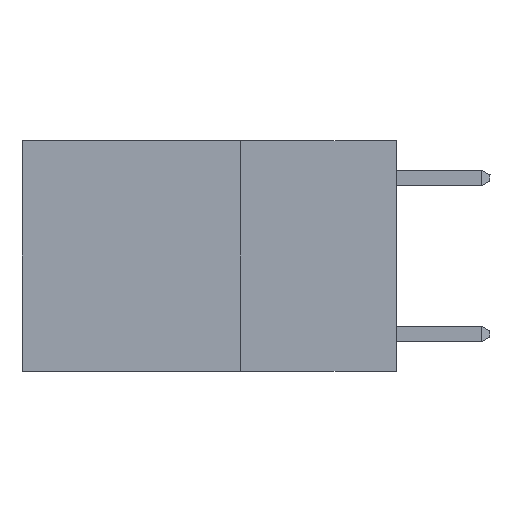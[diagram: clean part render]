
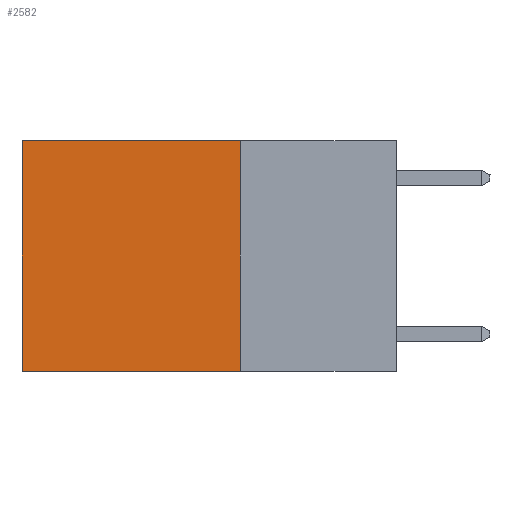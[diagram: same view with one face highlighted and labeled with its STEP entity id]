
A CAD part, left-side view. The second image highlights one B-rep face of the part: STEP entity #2582.
In plain terms, the highlighted planar face has unit normal (-1, 0, 0).
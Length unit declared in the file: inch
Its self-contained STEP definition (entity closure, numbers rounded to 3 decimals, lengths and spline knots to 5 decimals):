
#59 = LINE ( 'NONE', #6699, #10826 ) ;
#206 = CARTESIAN_POINT ( 'NONE',  ( 0.2625, 0.25, -0.37 ) ) ;
#1001 = DIRECTION ( 'NONE',  ( 0., 1., 0. ) ) ;
#1165 = CARTESIAN_POINT ( 'NONE',  ( 0.2625, 0.25, 0. ) ) ;
#1346 = EDGE_CURVE ( 'NONE', #12478, #9036, #5121, .T. ) ;
#1813 = CARTESIAN_POINT ( 'NONE',  ( 0.2625, 0.25, 0. ) ) ;
#2383 = VECTOR ( 'NONE', #9226, 39.37008 ) ;
#2495 = ORIENTED_EDGE ( 'NONE', *, *, #9617, .F. ) ;
#2582 = ADVANCED_FACE ( 'NONE', ( #8366 ), #13596, .F. ) ;
#3487 = EDGE_CURVE ( 'NONE', #10456, #3596, #10041, .T. ) ;
#3596 = VERTEX_POINT ( 'NONE', #206 ) ;
#3707 = LINE ( 'NONE', #1165, #13498 ) ;
#4572 = ORIENTED_EDGE ( 'NONE', *, *, #15252, .T. ) ;
#4646 = EDGE_LOOP ( 'NONE', ( #11900, #2495, #7291, #4572 ) ) ;
#5121 = LINE ( 'NONE', #14393, #2383 ) ;
#6699 = CARTESIAN_POINT ( 'NONE',  ( 0.2625, 0.25, -0.37 ) ) ;
#7075 = DIRECTION ( 'NONE',  ( 1., 0., 0. ) ) ;
#7291 = ORIENTED_EDGE ( 'NONE', *, *, #3487, .F. ) ;
#8366 = FACE_OUTER_BOUND ( 'NONE', #4646, .T. ) ;
#9036 = VERTEX_POINT ( 'NONE', #10096 ) ;
#9226 = DIRECTION ( 'NONE',  ( 0., 0., -1. ) ) ;
#9617 = EDGE_CURVE ( 'NONE', #3596, #9036, #59, .T. ) ;
#9729 = AXIS2_PLACEMENT_3D ( 'NONE', #1813, #7075, #16948 ) ;
#10041 = LINE ( 'NONE', #10207, #14725 ) ;
#10096 = CARTESIAN_POINT ( 'NONE',  ( 0.2625, 0.6, -0.37 ) ) ;
#10207 = CARTESIAN_POINT ( 'NONE',  ( 0.2625, 0.25, 0. ) ) ;
#10456 = VERTEX_POINT ( 'NONE', #13018 ) ;
#10732 = DIRECTION ( 'NONE',  ( 0., 1., 0. ) ) ;
#10826 = VECTOR ( 'NONE', #10732, 39.37008 ) ;
#11900 = ORIENTED_EDGE ( 'NONE', *, *, #1346, .T. ) ;
#12478 = VERTEX_POINT ( 'NONE', #14452 ) ;
#13018 = CARTESIAN_POINT ( 'NONE',  ( 0.2625, 0.25, 0. ) ) ;
#13498 = VECTOR ( 'NONE', #1001, 39.37008 ) ;
#13596 = PLANE ( 'NONE',  #9729 ) ;
#14393 = CARTESIAN_POINT ( 'NONE',  ( 0.2625, 0.6, 0. ) ) ;
#14452 = CARTESIAN_POINT ( 'NONE',  ( 0.2625, 0.6, 0. ) ) ;
#14725 = VECTOR ( 'NONE', #15283, 39.37008 ) ;
#15252 = EDGE_CURVE ( 'NONE', #10456, #12478, #3707, .T. ) ;
#15283 = DIRECTION ( 'NONE',  ( 0., 0., -1. ) ) ;
#16948 = DIRECTION ( 'NONE',  ( 0., 0., -1. ) ) ;
